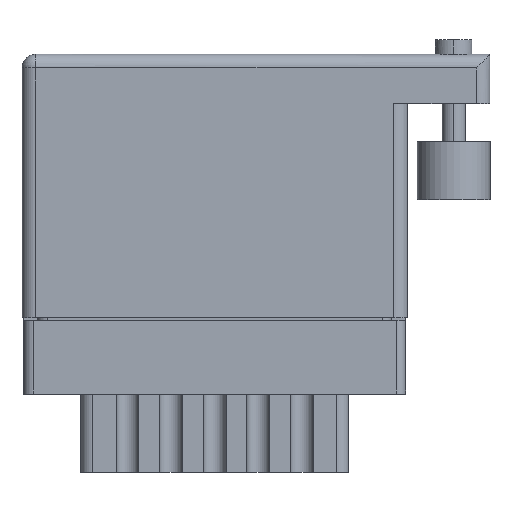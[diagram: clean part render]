
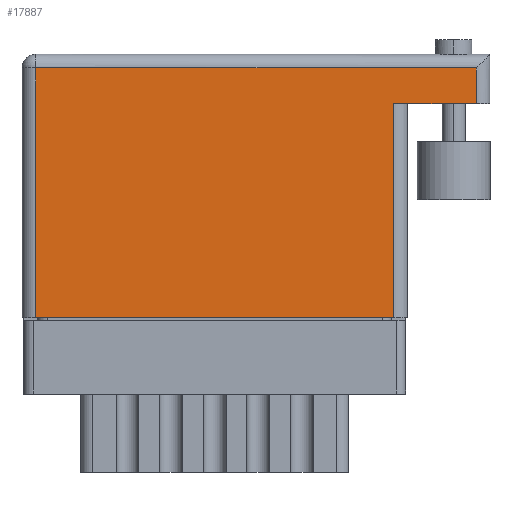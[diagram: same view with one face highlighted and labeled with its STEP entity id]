
A CAD part, front view. The second image highlights one B-rep face of the part: STEP entity #17887.
In plain terms, the highlighted face is planar.
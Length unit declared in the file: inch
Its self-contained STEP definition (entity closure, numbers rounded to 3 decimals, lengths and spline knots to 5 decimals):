
#251 = EDGE_CURVE ( 'NONE', #13491, #12579, #19864, .T. ) ;
#848 = CARTESIAN_POINT ( 'NONE',  ( 1.562, 0.736, 0. ) ) ;
#868 = CARTESIAN_POINT ( 'NONE',  ( 1.278, 0.736, 0. ) ) ;
#1644 = LINE ( 'NONE', #4004, #25368 ) ;
#1866 = DIRECTION ( 'NONE',  ( -1., 0., 0. ) ) ;
#2519 = VECTOR ( 'NONE', #14408, 39.37008 ) ;
#2790 = VECTOR ( 'NONE', #1866, 39.37008 ) ;
#2839 = LINE ( 'NONE', #868, #18339 ) ;
#4004 = CARTESIAN_POINT ( 'NONE',  ( 1.609, 0.736, 0. ) ) ;
#4700 = CARTESIAN_POINT ( 'NONE',  ( 0., 0., 0. ) ) ;
#5057 = CARTESIAN_POINT ( 'NONE',  ( 1.562, 0.906, 0. ) ) ;
#6104 = DIRECTION ( 'NONE',  ( -1., 0., 0. ) ) ;
#6211 = CARTESIAN_POINT ( 'NONE',  ( 0., 0.859, 0. ) ) ;
#6829 = ORIENTED_EDGE ( 'NONE', *, *, #251, .T. ) ;
#7953 = DIRECTION ( 'NONE',  ( -1., 0., 0. ) ) ;
#8074 = FACE_OUTER_BOUND ( 'NONE', #14821, .T. ) ;
#8141 = ORIENTED_EDGE ( 'NONE', *, *, #16541, .T. ) ;
#8419 = EDGE_CURVE ( 'NONE', #12579, #11012, #14012, .T. ) ;
#8875 = DIRECTION ( 'NONE',  ( 0., 1., 0. ) ) ;
#9124 = LINE ( 'NONE', #5057, #12067 ) ;
#10486 = CARTESIAN_POINT ( 'NONE',  ( 0.047, 0., 0. ) ) ;
#10585 = ORIENTED_EDGE ( 'NONE', *, *, #20157, .T. ) ;
#10841 = CARTESIAN_POINT ( 'NONE',  ( 0.047, 0., 0. ) ) ;
#11012 = VERTEX_POINT ( 'NONE', #10841 ) ;
#11088 = DIRECTION ( 'NONE',  ( 0., 1., 0. ) ) ;
#12067 = VECTOR ( 'NONE', #11088, 39.37008 ) ;
#12579 = VERTEX_POINT ( 'NONE', #14472 ) ;
#13283 = AXIS2_PLACEMENT_3D ( 'NONE', #24104, #17907, #6104 ) ;
#13491 = VERTEX_POINT ( 'NONE', #20728 ) ;
#14012 = LINE ( 'NONE', #10486, #2519 ) ;
#14061 = ORIENTED_EDGE ( 'NONE', *, *, #8419, .T. ) ;
#14062 = VERTEX_POINT ( 'NONE', #848 ) ;
#14408 = DIRECTION ( 'NONE',  ( 0., -1., 0. ) ) ;
#14472 = CARTESIAN_POINT ( 'NONE',  ( 0.047, 0.859, 0. ) ) ;
#14821 = EDGE_LOOP ( 'NONE', ( #10585, #23356, #23439, #8141, #6829, #14061 ) ) ;
#15835 = VERTEX_POINT ( 'NONE', #17722 ) ;
#16062 = PLANE ( 'NONE',  #13283 ) ;
#16541 = EDGE_CURVE ( 'NONE', #14062, #13491, #9124, .T. ) ;
#17722 = CARTESIAN_POINT ( 'NONE',  ( 1.278, 0.736, 0. ) ) ;
#17786 = VERTEX_POINT ( 'NONE', #18342 ) ;
#17887 = ADVANCED_FACE ( 'NONE', ( #8074 ), #16062, .F. ) ;
#17907 = DIRECTION ( 'NONE',  ( 0., 0., -1. ) ) ;
#18339 = VECTOR ( 'NONE', #8875, 39.37008 ) ;
#18342 = CARTESIAN_POINT ( 'NONE',  ( 1.278, 0., 0. ) ) ;
#19864 = LINE ( 'NONE', #6211, #2790 ) ;
#20157 = EDGE_CURVE ( 'NONE', #11012, #17786, #22703, .T. ) ;
#20278 = VECTOR ( 'NONE', #20723, 39.37008 ) ;
#20723 = DIRECTION ( 'NONE',  ( 1., 0., 0. ) ) ;
#20728 = CARTESIAN_POINT ( 'NONE',  ( 1.562, 0.859, 0. ) ) ;
#22440 = EDGE_CURVE ( 'NONE', #14062, #15835, #1644, .T. ) ;
#22703 = LINE ( 'NONE', #4700, #20278 ) ;
#23356 = ORIENTED_EDGE ( 'NONE', *, *, #25658, .T. ) ;
#23439 = ORIENTED_EDGE ( 'NONE', *, *, #22440, .F. ) ;
#24104 = CARTESIAN_POINT ( 'NONE',  ( 0., 0.906, 0. ) ) ;
#25368 = VECTOR ( 'NONE', #7953, 39.37008 ) ;
#25658 = EDGE_CURVE ( 'NONE', #17786, #15835, #2839, .T. ) ;
